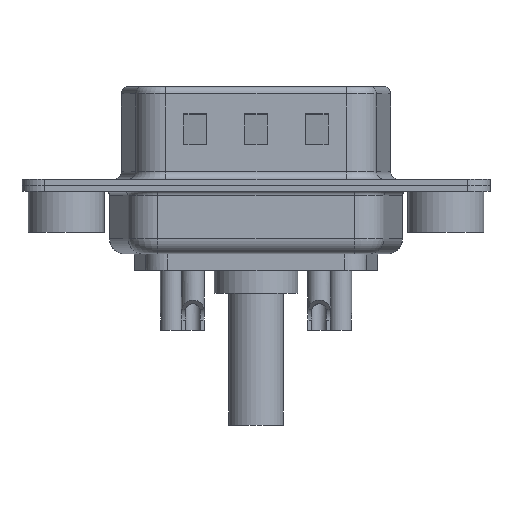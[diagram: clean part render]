
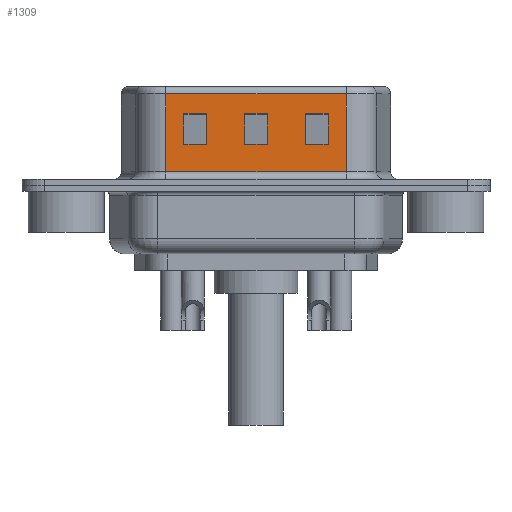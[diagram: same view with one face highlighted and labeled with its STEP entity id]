
A CAD part, front view. The second image highlights one B-rep face of the part: STEP entity #1309.
In plain terms, the highlighted planar face has unit normal (0, -1, 0).
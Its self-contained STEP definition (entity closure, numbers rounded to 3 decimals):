
#118 = DIRECTION ( 'NONE',  ( 0., 0., 1. ) ) ;
#196 = VECTOR ( 'NONE', #14351, 1000. ) ;
#231 = ORIENTED_EDGE ( 'NONE', *, *, #13798, .T. ) ;
#338 = EDGE_CURVE ( 'NONE', #8399, #5224, #9112, .T. ) ;
#527 = ORIENTED_EDGE ( 'NONE', *, *, #6318, .T. ) ;
#753 = CARTESIAN_POINT ( 'NONE',  ( 22.45, -4.58, 2.705 ) ) ;
#1263 = LINE ( 'NONE', #6929, #6749 ) ;
#1309 = ADVANCED_FACE ( 'NONE', ( #13589, #1536, #7382, #12871 ), #4494, .F. ) ;
#1340 = CARTESIAN_POINT ( 'NONE',  ( 6.55, -4.58, 6.02 ) ) ;
#1353 = VECTOR ( 'NONE', #5087, 1000. ) ;
#1365 = VERTEX_POINT ( 'NONE', #4590 ) ;
#1399 = DIRECTION ( 'NONE',  ( 0., 0., -1. ) ) ;
#1436 = ORIENTED_EDGE ( 'NONE', *, *, #9117, .T. ) ;
#1442 = EDGE_CURVE ( 'NONE', #2549, #11581, #11510, .T. ) ;
#1536 = FACE_BOUND ( 'NONE', #10653, .T. ) ;
#1608 = EDGE_CURVE ( 'NONE', #5907, #1365, #13402, .T. ) ;
#1698 = DIRECTION ( 'NONE',  ( 0., 1., 0. ) ) ;
#1808 = CARTESIAN_POINT ( 'NONE',  ( 7.75, -4.58, 4.705 ) ) ;
#1864 = VERTEX_POINT ( 'NONE', #3092 ) ;
#1954 = LINE ( 'NONE', #13172, #4539 ) ;
#2194 = EDGE_CURVE ( 'NONE', #7749, #12874, #6466, .T. ) ;
#2372 = LINE ( 'NONE', #11255, #10827 ) ;
#2482 = EDGE_LOOP ( 'NONE', ( #1436, #9345, #231, #11793 ) ) ;
#2549 = VERTEX_POINT ( 'NONE', #9765 ) ;
#2629 = EDGE_LOOP ( 'NONE', ( #3464, #13019, #7479, #8262 ) ) ;
#2872 = VERTEX_POINT ( 'NONE', #1808 ) ;
#2919 = EDGE_CURVE ( 'NONE', #10006, #2549, #14093, .T. ) ;
#3092 = CARTESIAN_POINT ( 'NONE',  ( 6.55, -4.58, 0.9 ) ) ;
#3339 = CARTESIAN_POINT ( 'NONE',  ( 14.45, -4.58, 2.705 ) ) ;
#3464 = ORIENTED_EDGE ( 'NONE', *, *, #338, .T. ) ;
#3582 = VECTOR ( 'NONE', #9561, 1000. ) ;
#3656 = ORIENTED_EDGE ( 'NONE', *, *, #2194, .T. ) ;
#3947 = CARTESIAN_POINT ( 'NONE',  ( 18.45, -4.58, 6.02 ) ) ;
#3949 = EDGE_CURVE ( 'NONE', #9716, #13953, #4088, .T. ) ;
#4069 = CARTESIAN_POINT ( 'NONE',  ( 13.25, -4.58, 2.705 ) ) ;
#4088 = LINE ( 'NONE', #4754, #13182 ) ;
#4178 = LINE ( 'NONE', #13299, #7431 ) ;
#4402 = DIRECTION ( 'NONE',  ( 1., 0., 0. ) ) ;
#4494 = PLANE ( 'NONE',  #8114 ) ;
#4504 = DIRECTION ( 'NONE',  ( 0., 0., -1. ) ) ;
#4516 = CARTESIAN_POINT ( 'NONE',  ( 15.75, -4.58, 2.705 ) ) ;
#4539 = VECTOR ( 'NONE', #14298, 1000. ) ;
#4590 = CARTESIAN_POINT ( 'NONE',  ( 11.75, -4.58, 4.705 ) ) ;
#4708 = ORIENTED_EDGE ( 'NONE', *, *, #11879, .F. ) ;
#4737 = DIRECTION ( 'NONE',  ( 0., 0., 1. ) ) ;
#4754 = CARTESIAN_POINT ( 'NONE',  ( 13.25, -4.58, 6.52 ) ) ;
#4804 = DIRECTION ( 'NONE',  ( 0., 0., -1. ) ) ;
#4835 = VECTOR ( 'NONE', #14077, 1000. ) ;
#4973 = DIRECTION ( 'NONE',  ( -1., 0., 0. ) ) ;
#5086 = VERTEX_POINT ( 'NONE', #7336 ) ;
#5087 = DIRECTION ( 'NONE',  ( 0., 0., 1. ) ) ;
#5100 = EDGE_CURVE ( 'NONE', #2872, #8399, #12120, .T. ) ;
#5127 = ORIENTED_EDGE ( 'NONE', *, *, #12022, .T. ) ;
#5224 = VERTEX_POINT ( 'NONE', #13392 ) ;
#5513 = DIRECTION ( 'NONE',  ( 0., 0., -1. ) ) ;
#5623 = ORIENTED_EDGE ( 'NONE', *, *, #2919, .T. ) ;
#5833 = EDGE_CURVE ( 'NONE', #13940, #2872, #1263, .T. ) ;
#5907 = VERTEX_POINT ( 'NONE', #5909 ) ;
#5909 = CARTESIAN_POINT ( 'NONE',  ( 11.75, -4.58, 2.705 ) ) ;
#5955 = EDGE_LOOP ( 'NONE', ( #4708, #3656, #9106, #527 ) ) ;
#6318 = EDGE_CURVE ( 'NONE', #1864, #12456, #1954, .T. ) ;
#6466 = LINE ( 'NONE', #3947, #3582 ) ;
#6595 = CARTESIAN_POINT ( 'NONE',  ( 17.25, -4.58, 4.705 ) ) ;
#6637 = CARTESIAN_POINT ( 'NONE',  ( 18.45, -4.58, 6.52 ) ) ;
#6749 = VECTOR ( 'NONE', #4737, 1000. ) ;
#6929 = CARTESIAN_POINT ( 'NONE',  ( 7.75, -4.58, 6.52 ) ) ;
#7336 = CARTESIAN_POINT ( 'NONE',  ( 15.75, -4.58, 4.705 ) ) ;
#7382 = FACE_BOUND ( 'NONE', #2482, .T. ) ;
#7412 = CARTESIAN_POINT ( 'NONE',  ( 14.45, -4.58, 4.705 ) ) ;
#7431 = VECTOR ( 'NONE', #14419, 1000. ) ;
#7479 = ORIENTED_EDGE ( 'NONE', *, *, #5833, .T. ) ;
#7749 = VERTEX_POINT ( 'NONE', #8062 ) ;
#7872 = LINE ( 'NONE', #7938, #13381 ) ;
#7938 = CARTESIAN_POINT ( 'NONE',  ( 6.55, -4.58, 6.52 ) ) ;
#8062 = CARTESIAN_POINT ( 'NONE',  ( 18.45, -4.58, 6.02 ) ) ;
#8114 = AXIS2_PLACEMENT_3D ( 'NONE', #6637, #1698, #8170 ) ;
#8170 = DIRECTION ( 'NONE',  ( 0., 0., 1. ) ) ;
#8262 = ORIENTED_EDGE ( 'NONE', *, *, #5100, .T. ) ;
#8399 = VERTEX_POINT ( 'NONE', #11309 ) ;
#8495 = CARTESIAN_POINT ( 'NONE',  ( 17.25, -4.58, 6.52 ) ) ;
#8539 = LINE ( 'NONE', #10505, #12979 ) ;
#8578 = CARTESIAN_POINT ( 'NONE',  ( 11.75, -4.58, 6.52 ) ) ;
#8599 = VECTOR ( 'NONE', #12824, 1000. ) ;
#8890 = VECTOR ( 'NONE', #9097, 1000. ) ;
#9097 = DIRECTION ( 'NONE',  ( 1., 0., 0. ) ) ;
#9106 = ORIENTED_EDGE ( 'NONE', *, *, #12043, .T. ) ;
#9112 = LINE ( 'NONE', #13560, #196 ) ;
#9117 = EDGE_CURVE ( 'NONE', #1365, #9716, #4178, .T. ) ;
#9345 = ORIENTED_EDGE ( 'NONE', *, *, #3949, .T. ) ;
#9561 = DIRECTION ( 'NONE',  ( -1., 0., 0. ) ) ;
#9571 = EDGE_CURVE ( 'NONE', #5224, #13940, #13259, .T. ) ;
#9716 = VERTEX_POINT ( 'NONE', #11536 ) ;
#9765 = CARTESIAN_POINT ( 'NONE',  ( 17.25, -4.58, 2.705 ) ) ;
#9973 = LINE ( 'NONE', #13216, #12520 ) ;
#10006 = VERTEX_POINT ( 'NONE', #6595 ) ;
#10505 = CARTESIAN_POINT ( 'NONE',  ( 18.45, -4.58, 2.705 ) ) ;
#10599 = EDGE_CURVE ( 'NONE', #5086, #10006, #14284, .T. ) ;
#10653 = EDGE_LOOP ( 'NONE', ( #5623, #12322, #5127, #12730 ) ) ;
#10827 = VECTOR ( 'NONE', #118, 1000. ) ;
#11255 = CARTESIAN_POINT ( 'NONE',  ( 15.75, -4.58, 6.52 ) ) ;
#11309 = CARTESIAN_POINT ( 'NONE',  ( 9.25, -4.58, 4.705 ) ) ;
#11498 = VECTOR ( 'NONE', #4804, 1000. ) ;
#11510 = LINE ( 'NONE', #753, #8599 ) ;
#11536 = CARTESIAN_POINT ( 'NONE',  ( 13.25, -4.58, 4.705 ) ) ;
#11581 = VERTEX_POINT ( 'NONE', #4516 ) ;
#11704 = VECTOR ( 'NONE', #4402, 1000. ) ;
#11793 = ORIENTED_EDGE ( 'NONE', *, *, #1608, .T. ) ;
#11879 = EDGE_CURVE ( 'NONE', #7749, #12456, #9973, .T. ) ;
#12022 = EDGE_CURVE ( 'NONE', #11581, #5086, #2372, .T. ) ;
#12043 = EDGE_CURVE ( 'NONE', #12874, #1864, #7872, .T. ) ;
#12077 = CARTESIAN_POINT ( 'NONE',  ( 22.45, -4.58, 4.705 ) ) ;
#12120 = LINE ( 'NONE', #7412, #8890 ) ;
#12322 = ORIENTED_EDGE ( 'NONE', *, *, #1442, .T. ) ;
#12456 = VERTEX_POINT ( 'NONE', #13057 ) ;
#12520 = VECTOR ( 'NONE', #5513, 1000. ) ;
#12730 = ORIENTED_EDGE ( 'NONE', *, *, #10599, .T. ) ;
#12824 = DIRECTION ( 'NONE',  ( -1., 0., 0. ) ) ;
#12871 = FACE_OUTER_BOUND ( 'NONE', #5955, .T. ) ;
#12874 = VERTEX_POINT ( 'NONE', #1340 ) ;
#12887 = CARTESIAN_POINT ( 'NONE',  ( 7.75, -4.58, 2.705 ) ) ;
#12979 = VECTOR ( 'NONE', #4973, 1000. ) ;
#13019 = ORIENTED_EDGE ( 'NONE', *, *, #9571, .T. ) ;
#13057 = CARTESIAN_POINT ( 'NONE',  ( 18.45, -4.58, 0.9 ) ) ;
#13172 = CARTESIAN_POINT ( 'NONE',  ( 18.45, -4.58, 0.9 ) ) ;
#13182 = VECTOR ( 'NONE', #4504, 1000. ) ;
#13216 = CARTESIAN_POINT ( 'NONE',  ( 18.45, -4.58, 6.52 ) ) ;
#13259 = LINE ( 'NONE', #3339, #4835 ) ;
#13299 = CARTESIAN_POINT ( 'NONE',  ( 18.45, -4.58, 4.705 ) ) ;
#13381 = VECTOR ( 'NONE', #1399, 1000. ) ;
#13392 = CARTESIAN_POINT ( 'NONE',  ( 9.25, -4.58, 2.705 ) ) ;
#13402 = LINE ( 'NONE', #8578, #1353 ) ;
#13560 = CARTESIAN_POINT ( 'NONE',  ( 9.25, -4.58, 6.52 ) ) ;
#13589 = FACE_BOUND ( 'NONE', #2629, .T. ) ;
#13798 = EDGE_CURVE ( 'NONE', #13953, #5907, #8539, .T. ) ;
#13940 = VERTEX_POINT ( 'NONE', #12887 ) ;
#13953 = VERTEX_POINT ( 'NONE', #4069 ) ;
#14077 = DIRECTION ( 'NONE',  ( -1., 0., 0. ) ) ;
#14093 = LINE ( 'NONE', #8495, #11498 ) ;
#14284 = LINE ( 'NONE', #12077, #11704 ) ;
#14298 = DIRECTION ( 'NONE',  ( 1., 0., 0. ) ) ;
#14351 = DIRECTION ( 'NONE',  ( 0., 0., -1. ) ) ;
#14419 = DIRECTION ( 'NONE',  ( 1., 0., 0. ) ) ;
